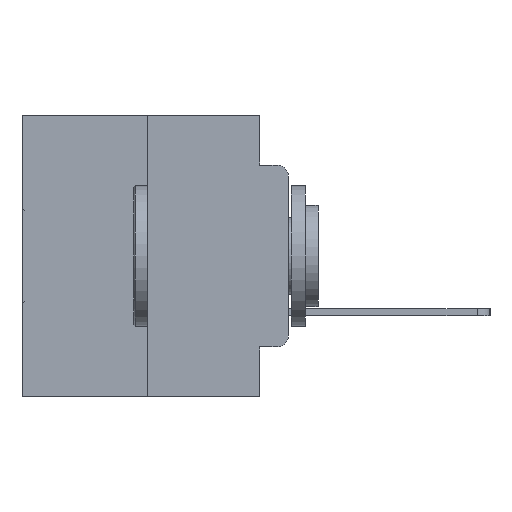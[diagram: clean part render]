
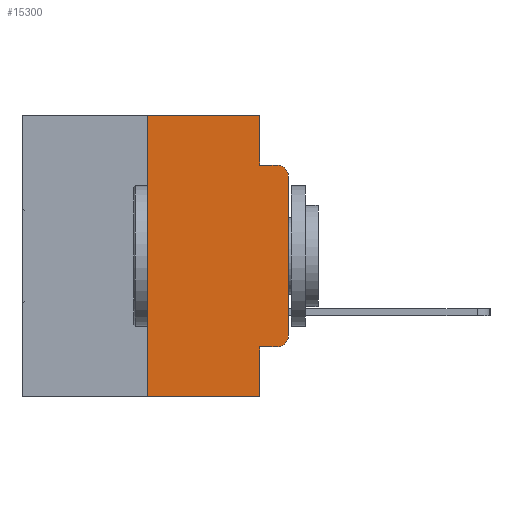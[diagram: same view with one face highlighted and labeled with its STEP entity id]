
A CAD part, left-side view. The second image highlights one B-rep face of the part: STEP entity #15300.
In plain terms, the highlighted planar face has unit normal (-1, 0, 0).
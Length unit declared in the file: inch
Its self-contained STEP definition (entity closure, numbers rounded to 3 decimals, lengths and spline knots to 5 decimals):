
#165 = VERTEX_POINT ( 'NONE', #26989 ) ;
#335 = LINE ( 'NONE', #5151, #18653 ) ;
#1078 = ORIENTED_EDGE ( 'NONE', *, *, #7000, .F. ) ;
#1985 = AXIS2_PLACEMENT_3D ( 'NONE', #9410, #25740, #11835 ) ;
#2608 = VECTOR ( 'NONE', #18393, 39.37008 ) ;
#2836 = VECTOR ( 'NONE', #26653, 39.37008 ) ;
#2876 = CARTESIAN_POINT ( 'NONE',  ( 0., 0.051, -0.0885 ) ) ;
#3350 = ORIENTED_EDGE ( 'NONE', *, *, #27312, .T. ) ;
#3708 = AXIS2_PLACEMENT_3D ( 'NONE', #28588, #10124, #26418 ) ;
#3756 = EDGE_CURVE ( 'NONE', #5893, #4020, #9229, .T. ) ;
#3939 = VERTEX_POINT ( 'NONE', #3979 ) ;
#3979 = CARTESIAN_POINT ( 'NONE',  ( 0., 0.051, 0. ) ) ;
#4020 = VERTEX_POINT ( 'NONE', #20886 ) ;
#4379 = VERTEX_POINT ( 'NONE', #22152 ) ;
#4487 = CARTESIAN_POINT ( 'NONE',  ( 0., 0.051, -0.4115 ) ) ;
#4513 = CARTESIAN_POINT ( 'NONE',  ( 0., 0., -0.1085 ) ) ;
#4929 = CIRCLE ( 'NONE', #16218, 0.02 ) ;
#5151 = CARTESIAN_POINT ( 'NONE',  ( 0., 0.473, 0. ) ) ;
#5361 = EDGE_CURVE ( 'NONE', #5893, #4379, #10244, .T. ) ;
#5614 = ORIENTED_EDGE ( 'NONE', *, *, #21252, .T. ) ;
#5893 = VERTEX_POINT ( 'NONE', #4487 ) ;
#6526 = VECTOR ( 'NONE', #24216, 39.37008 ) ;
#7000 = EDGE_CURVE ( 'NONE', #13821, #20005, #9017, .T. ) ;
#7101 = CARTESIAN_POINT ( 'NONE',  ( 0., 0.473, -0.5 ) ) ;
#7161 = EDGE_LOOP ( 'NONE', ( #3350, #5614, #26507, #17193, #17917, #1078, #22982, #12025, #19756, #8649 ) ) ;
#7571 = DIRECTION ( 'NONE',  ( 0., -1., 0. ) ) ;
#8649 = ORIENTED_EDGE ( 'NONE', *, *, #29427, .T. ) ;
#8769 = VERTEX_POINT ( 'NONE', #27584 ) ;
#9017 = LINE ( 'NONE', #16046, #2608 ) ;
#9045 = CARTESIAN_POINT ( 'NONE',  ( 0., 0.25, -0.5 ) ) ;
#9229 = LINE ( 'NONE', #10385, #2836 ) ;
#9410 = CARTESIAN_POINT ( 'NONE',  ( 0., 0.02, -0.1085 ) ) ;
#9664 = DIRECTION ( 'NONE',  ( -1., 0., 0. ) ) ;
#10001 = CARTESIAN_POINT ( 'NONE',  ( 0., 0.051, 0. ) ) ;
#10124 = DIRECTION ( 'NONE',  ( 1., 0., 0. ) ) ;
#10244 = LINE ( 'NONE', #23885, #22007 ) ;
#10385 = CARTESIAN_POINT ( 'NONE',  ( 0., 0.051, -0.4115 ) ) ;
#10571 = VECTOR ( 'NONE', #14820, 39.37008 ) ;
#11806 = EDGE_CURVE ( 'NONE', #3939, #8769, #12900, .T. ) ;
#11835 = DIRECTION ( 'NONE',  ( 0., 0., -1. ) ) ;
#12025 = ORIENTED_EDGE ( 'NONE', *, *, #5361, .F. ) ;
#12217 = VERTEX_POINT ( 'NONE', #21016 ) ;
#12259 = VERTEX_POINT ( 'NONE', #4513 ) ;
#12419 = DIRECTION ( 'NONE',  ( 0., 0., -1. ) ) ;
#12844 = LINE ( 'NONE', #2876, #10571 ) ;
#12900 = LINE ( 'NONE', #10001, #24501 ) ;
#13231 = EDGE_CURVE ( 'NONE', #13821, #4379, #28002, .T. ) ;
#13406 = EDGE_CURVE ( 'NONE', #8769, #12217, #12844, .T. ) ;
#13821 = VERTEX_POINT ( 'NONE', #9045 ) ;
#14052 = EDGE_CURVE ( 'NONE', #20005, #3939, #335, .T. ) ;
#14316 = DIRECTION ( 'NONE',  ( 0., -1., 0. ) ) ;
#14671 = DIRECTION ( 'NONE',  ( 0., 0., -1. ) ) ;
#14820 = DIRECTION ( 'NONE',  ( 0., -1., 0. ) ) ;
#15300 = ADVANCED_FACE ( 'NONE', ( #19170 ), #24125, .F. ) ;
#16046 = CARTESIAN_POINT ( 'NONE',  ( 0., 0.25, 0. ) ) ;
#16218 = AXIS2_PLACEMENT_3D ( 'NONE', #23681, #9664, #25972 ) ;
#17193 = ORIENTED_EDGE ( 'NONE', *, *, #11806, .F. ) ;
#17917 = ORIENTED_EDGE ( 'NONE', *, *, #14052, .F. ) ;
#18393 = DIRECTION ( 'NONE',  ( 0., 0., 1. ) ) ;
#18653 = VECTOR ( 'NONE', #7571, 39.37008 ) ;
#19170 = FACE_OUTER_BOUND ( 'NONE', #7161, .T. ) ;
#19756 = ORIENTED_EDGE ( 'NONE', *, *, #3756, .T. ) ;
#20005 = VERTEX_POINT ( 'NONE', #28845 ) ;
#20304 = CIRCLE ( 'NONE', #1985, 0.02 ) ;
#20886 = CARTESIAN_POINT ( 'NONE',  ( 0., 0.02, -0.4115 ) ) ;
#21016 = CARTESIAN_POINT ( 'NONE',  ( 0., 0.02, -0.0885 ) ) ;
#21252 = EDGE_CURVE ( 'NONE', #12259, #12217, #20304, .T. ) ;
#22007 = VECTOR ( 'NONE', #14671, 39.37008 ) ;
#22152 = CARTESIAN_POINT ( 'NONE',  ( 0., 0.051, -0.5 ) ) ;
#22689 = VECTOR ( 'NONE', #14316, 39.37008 ) ;
#22982 = ORIENTED_EDGE ( 'NONE', *, *, #13231, .T. ) ;
#23681 = CARTESIAN_POINT ( 'NONE',  ( 0., 0.02, -0.3915 ) ) ;
#23885 = CARTESIAN_POINT ( 'NONE',  ( 0., 0.051, 0. ) ) ;
#24125 = PLANE ( 'NONE',  #3708 ) ;
#24216 = DIRECTION ( 'NONE',  ( 0., 0., 1. ) ) ;
#24501 = VECTOR ( 'NONE', #12419, 39.37008 ) ;
#25201 = LINE ( 'NONE', #26503, #6526 ) ;
#25740 = DIRECTION ( 'NONE',  ( -1., 0., 0. ) ) ;
#25972 = DIRECTION ( 'NONE',  ( 0., 0., -1. ) ) ;
#26418 = DIRECTION ( 'NONE',  ( 0., 0., -1. ) ) ;
#26503 = CARTESIAN_POINT ( 'NONE',  ( 0., 0., 0. ) ) ;
#26507 = ORIENTED_EDGE ( 'NONE', *, *, #13406, .F. ) ;
#26653 = DIRECTION ( 'NONE',  ( 0., -1., 0. ) ) ;
#26989 = CARTESIAN_POINT ( 'NONE',  ( 0., 0., -0.3915 ) ) ;
#27312 = EDGE_CURVE ( 'NONE', #165, #12259, #25201, .T. ) ;
#27584 = CARTESIAN_POINT ( 'NONE',  ( 0., 0.051, -0.0885 ) ) ;
#28002 = LINE ( 'NONE', #7101, #22689 ) ;
#28588 = CARTESIAN_POINT ( 'NONE',  ( 0., 0.473, 0. ) ) ;
#28845 = CARTESIAN_POINT ( 'NONE',  ( 0., 0.25, 0. ) ) ;
#29427 = EDGE_CURVE ( 'NONE', #4020, #165, #4929, .T. ) ;
